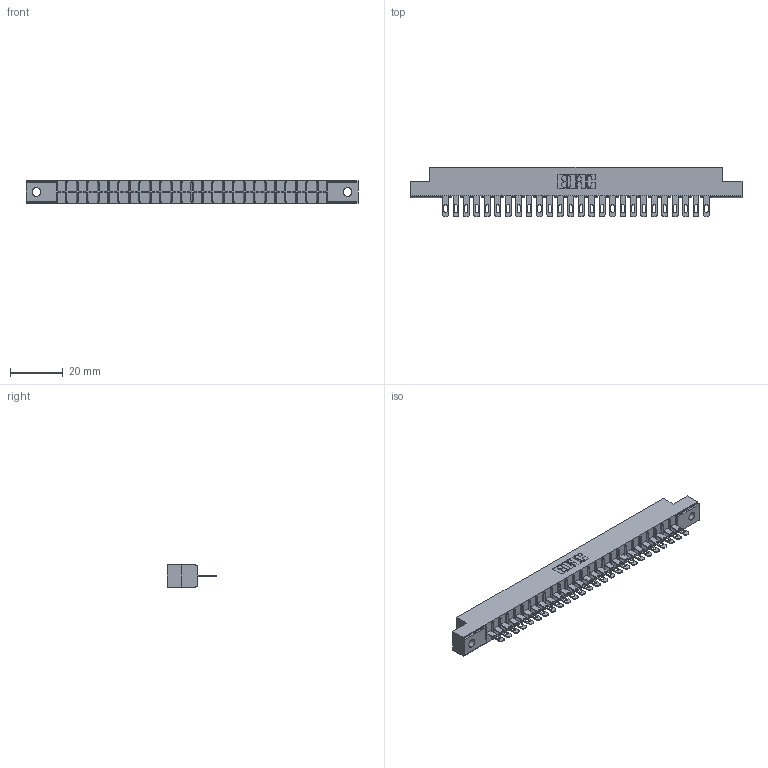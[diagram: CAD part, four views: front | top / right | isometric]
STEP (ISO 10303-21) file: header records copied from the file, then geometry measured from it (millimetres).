
FILE_DESCRIPTION (( 'STEP AP203' ), '1' );
FILE_NAME ('356-026-500-102.STEP', '2018-08-01T20:20:46', ( '' ), ( '' ), 'SwSTEP 2.0', 'SolidWorks 2016', '' );
FILE_SCHEMA (( 'CONFIG_CONTROL_DESIGN' ));
Length unit declared in the file: inch
Products named in the file (3): 356-026-500-102; 306 Part_.128 Dia; 306-290-001_100
Assembly tree (27 placements, depth 2):
  356-026-500-102
    306 Part_.128 Dia
    306-290-001_100  x26
Bounding box: 126.03 x 18.87 x 8.71 mm (x, y, z)
Volume: 8680.4 mm3; surface area: 13121.7 mm2
Topology: 27 solids, 27 shells, 2092 faces, 5906 edges, 3796 vertices
Faces by surface type: plane 1368, cylinder 620, sphere 104
Entity records: 26485 total; most frequent: CARTESIAN_POINT 4445, ORIENTED_EDGE 4404, DIRECTION 4386, EDGE_CURVE 2202, VECTOR 1712, LINE 1712, VERTEX_POINT 1396, AXIS2_PLACEMENT_3D 1337
